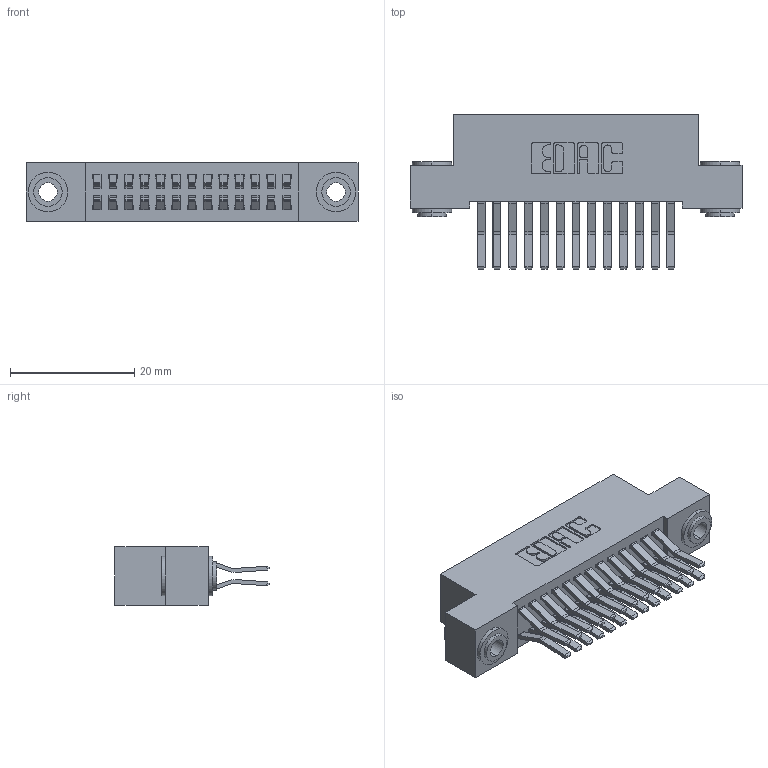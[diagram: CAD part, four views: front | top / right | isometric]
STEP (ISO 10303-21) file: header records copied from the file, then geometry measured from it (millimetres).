
FILE_DESCRIPTION (( 'STEP AP203' ), '1' );
FILE_NAME ('392-026-560-203.STEP', '2019-10-07T11:43:59', ( '' ), ( '' ), 'SwSTEP 2.0', 'SolidWorks 2016', '' );
FILE_SCHEMA (( 'CONFIG_CONTROL_DESIGN' ));
Length unit declared in the file: inch
Products named in the file (4): 345-292-001_560 Tail; 342 Part_.156 TH; 342-250-002_345-250-002-102; 392-026-560-203
Assembly tree (29 placements, depth 2):
  392-026-560-203
    342 Part_.156 TH
    345-292-001_560 Tail  x26
    342-250-002_345-250-002-102  x2
Bounding box: 53.34 x 24.78 x 9.4 mm (x, y, z)
Volume: 4848.8 mm3; surface area: 7801.5 mm2
Topology: 29 solids, 29 shells, 1552 faces, 4561 edges, 3002 vertices
Faces by surface type: plane 1012, cylinder 532, cone 8
Entity records: 12720 total; most frequent: CARTESIAN_POINT 2117, ORIENTED_EDGE 2046, DIRECTION 1897, EDGE_CURVE 1023, LINE 867, VECTOR 867, VERTEX_POINT 678, AXIS2_PLACEMENT_3D 515
